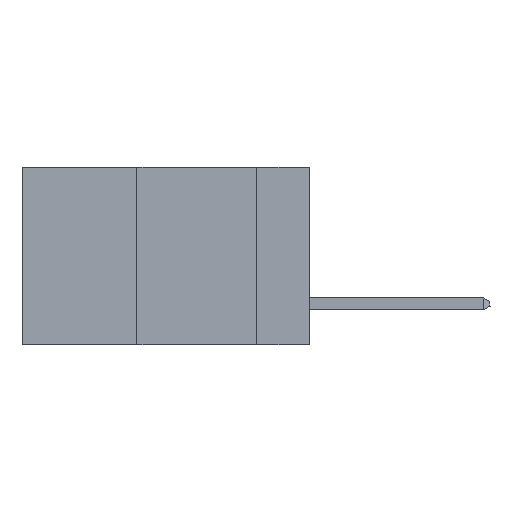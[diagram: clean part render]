
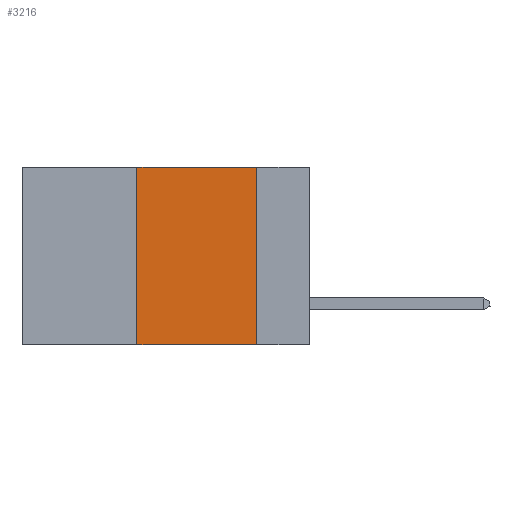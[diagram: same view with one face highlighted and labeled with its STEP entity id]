
A CAD part, left-side view. The second image highlights one B-rep face of the part: STEP entity #3216.
In plain terms, the highlighted planar face has unit normal (-1, 0, 0).
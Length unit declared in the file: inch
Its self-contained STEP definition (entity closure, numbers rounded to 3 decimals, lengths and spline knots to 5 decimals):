
#295 = EDGE_CURVE ( 'NONE', #12748, #24918, #2130, .T. ) ;
#1655 = CARTESIAN_POINT ( 'NONE',  ( 0., 0.6, 0. ) ) ;
#2130 = LINE ( 'NONE', #3723, #6537 ) ;
#3066 = CARTESIAN_POINT ( 'NONE',  ( 0., 0.36, 0. ) ) ;
#3216 = ADVANCED_FACE ( 'NONE', ( #21002 ), #22266, .F. ) ;
#3503 = ORIENTED_EDGE ( 'NONE', *, *, #15454, .F. ) ;
#3723 = CARTESIAN_POINT ( 'NONE',  ( 0., 0.6, -0.37 ) ) ;
#3799 = LINE ( 'NONE', #24798, #26797 ) ;
#4217 = ORIENTED_EDGE ( 'NONE', *, *, #295, .T. ) ;
#4237 = ORIENTED_EDGE ( 'NONE', *, *, #4958, .F. ) ;
#4272 = LINE ( 'NONE', #6882, #21201 ) ;
#4958 = EDGE_CURVE ( 'NONE', #22832, #18256, #27606, .T. ) ;
#6537 = VECTOR ( 'NONE', #19239, 39.37008 ) ;
#6882 = CARTESIAN_POINT ( 'NONE',  ( 0., 0.11, 0. ) ) ;
#12748 = VERTEX_POINT ( 'NONE', #19404 ) ;
#15454 = EDGE_CURVE ( 'NONE', #12748, #22832, #3799, .T. ) ;
#17669 = DIRECTION ( 'NONE',  ( 0., 0., -1. ) ) ;
#18256 = VERTEX_POINT ( 'NONE', #26812 ) ;
#18465 = EDGE_LOOP ( 'NONE', ( #20435, #4237, #3503, #4217 ) ) ;
#19239 = DIRECTION ( 'NONE',  ( 0., -1., 0. ) ) ;
#19404 = CARTESIAN_POINT ( 'NONE',  ( 0., 0.36, -0.37 ) ) ;
#20185 = AXIS2_PLACEMENT_3D ( 'NONE', #22364, #26412, #26602 ) ;
#20435 = ORIENTED_EDGE ( 'NONE', *, *, #25805, .F. ) ;
#20546 = VECTOR ( 'NONE', #27637, 39.37008 ) ;
#21002 = FACE_OUTER_BOUND ( 'NONE', #18465, .T. ) ;
#21201 = VECTOR ( 'NONE', #17669, 39.37008 ) ;
#22266 = PLANE ( 'NONE',  #20185 ) ;
#22364 = CARTESIAN_POINT ( 'NONE',  ( 0., 0.6, 0. ) ) ;
#22832 = VERTEX_POINT ( 'NONE', #3066 ) ;
#24619 = DIRECTION ( 'NONE',  ( 0., 0., 1. ) ) ;
#24798 = CARTESIAN_POINT ( 'NONE',  ( 0., 0.36, 0. ) ) ;
#24918 = VERTEX_POINT ( 'NONE', #25710 ) ;
#25710 = CARTESIAN_POINT ( 'NONE',  ( 0., 0.11, -0.37 ) ) ;
#25805 = EDGE_CURVE ( 'NONE', #18256, #24918, #4272, .T. ) ;
#26412 = DIRECTION ( 'NONE',  ( 1., 0., 0. ) ) ;
#26602 = DIRECTION ( 'NONE',  ( 0., 0., -1. ) ) ;
#26797 = VECTOR ( 'NONE', #24619, 39.37008 ) ;
#26812 = CARTESIAN_POINT ( 'NONE',  ( 0., 0.11, 0. ) ) ;
#27606 = LINE ( 'NONE', #1655, #20546 ) ;
#27637 = DIRECTION ( 'NONE',  ( 0., -1., 0. ) ) ;
